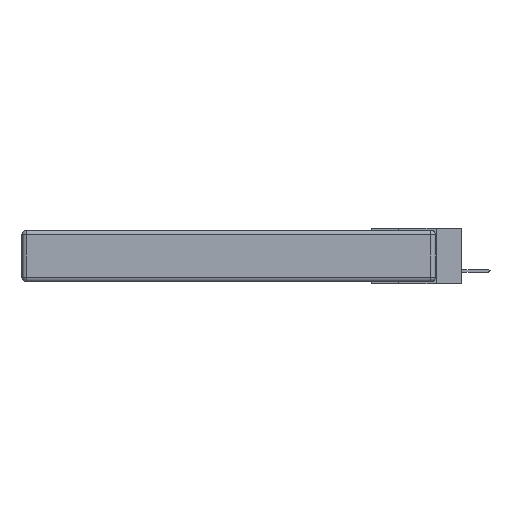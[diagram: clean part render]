
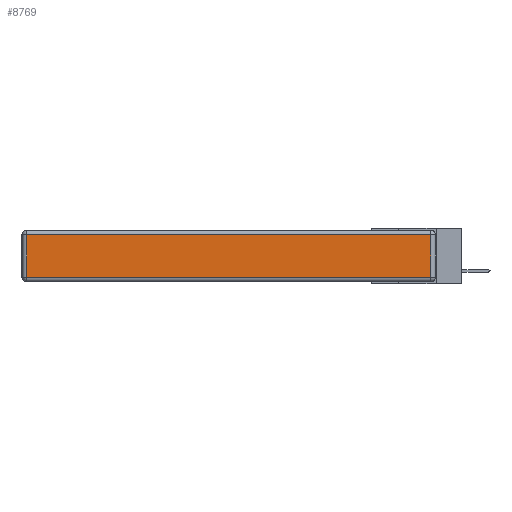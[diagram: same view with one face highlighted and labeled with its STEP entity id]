
A CAD part, left-side view. The second image highlights one B-rep face of the part: STEP entity #8769.
In plain terms, the highlighted planar face has unit normal (-1, 0, 0).
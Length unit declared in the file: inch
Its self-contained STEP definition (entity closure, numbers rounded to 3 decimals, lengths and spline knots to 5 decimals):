
#1059 = EDGE_CURVE ( 'NONE', #27005, #31603, #31013, .T. ) ;
#2749 = ORIENTED_EDGE ( 'NONE', *, *, #14004, .T. ) ;
#4126 = ORIENTED_EDGE ( 'NONE', *, *, #7988, .T. ) ;
#4437 = CARTESIAN_POINT ( 'NONE',  ( 0., 2.75, -0.03 ) ) ;
#4438 = DIRECTION ( 'NONE',  ( 0., 0., 1. ) ) ;
#4641 = DIRECTION ( 'NONE',  ( 0., 1., 0. ) ) ;
#6961 = CARTESIAN_POINT ( 'NONE',  ( 0., 0.03, -0.03 ) ) ;
#7333 = CARTESIAN_POINT ( 'NONE',  ( 0., 0., -0.313 ) ) ;
#7988 = EDGE_CURVE ( 'NONE', #31603, #26281, #17016, .T. ) ;
#8769 = ADVANCED_FACE ( 'NONE', ( #24815 ), #28230, .T. ) ;
#9059 = CARTESIAN_POINT ( 'NONE',  ( 0., 2.72, -0.03 ) ) ;
#9566 = CARTESIAN_POINT ( 'NONE',  ( 0., 0.03, -0.343 ) ) ;
#10265 = VERTEX_POINT ( 'NONE', #21424 ) ;
#11319 = AXIS2_PLACEMENT_3D ( 'NONE', #27802, #18258, #18145 ) ;
#11845 = DIRECTION ( 'NONE',  ( 0., -1., 0. ) ) ;
#12749 = VECTOR ( 'NONE', #4641, 39.37008 ) ;
#13460 = VECTOR ( 'NONE', #4438, 39.37008 ) ;
#14004 = EDGE_CURVE ( 'NONE', #10265, #27005, #30408, .T. ) ;
#15186 = ORIENTED_EDGE ( 'NONE', *, *, #1059, .T. ) ;
#15846 = LINE ( 'NONE', #19669, #19281 ) ;
#16356 = VECTOR ( 'NONE', #11845, 39.37008 ) ;
#16581 = CARTESIAN_POINT ( 'NONE',  ( 0., 0.03, -0.313 ) ) ;
#17016 = LINE ( 'NONE', #4437, #12749 ) ;
#18145 = DIRECTION ( 'NONE',  ( 0., 0., 1. ) ) ;
#18258 = DIRECTION ( 'NONE',  ( -1., 0., 0. ) ) ;
#19281 = VECTOR ( 'NONE', #29726, 39.37008 ) ;
#19625 = EDGE_LOOP ( 'NONE', ( #2749, #15186, #4126, #26023 ) ) ;
#19669 = CARTESIAN_POINT ( 'NONE',  ( 0., 2.72, -0.343 ) ) ;
#21424 = CARTESIAN_POINT ( 'NONE',  ( 0., 2.72, -0.313 ) ) ;
#24815 = FACE_OUTER_BOUND ( 'NONE', #19625, .T. ) ;
#26023 = ORIENTED_EDGE ( 'NONE', *, *, #30881, .T. ) ;
#26281 = VERTEX_POINT ( 'NONE', #9059 ) ;
#27005 = VERTEX_POINT ( 'NONE', #16581 ) ;
#27802 = CARTESIAN_POINT ( 'NONE',  ( 0., 0., -0.343 ) ) ;
#28230 = PLANE ( 'NONE',  #11319 ) ;
#29726 = DIRECTION ( 'NONE',  ( 0., 0., -1. ) ) ;
#30408 = LINE ( 'NONE', #7333, #16356 ) ;
#30881 = EDGE_CURVE ( 'NONE', #26281, #10265, #15846, .T. ) ;
#31013 = LINE ( 'NONE', #9566, #13460 ) ;
#31603 = VERTEX_POINT ( 'NONE', #6961 ) ;
